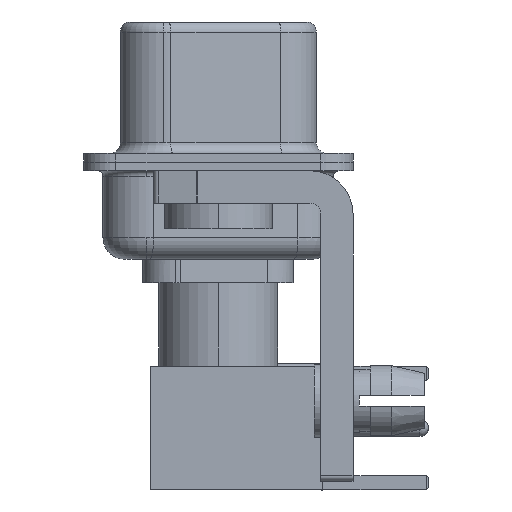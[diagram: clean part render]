
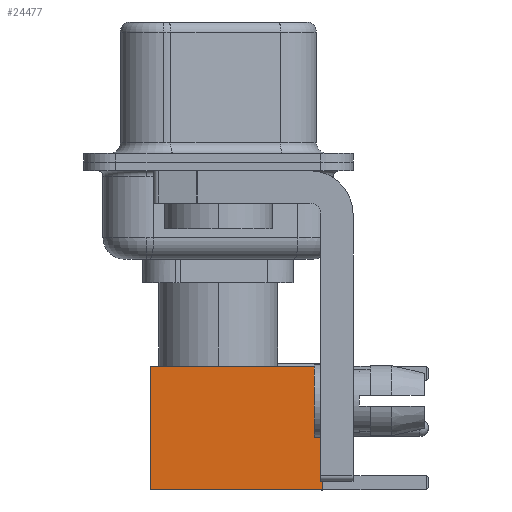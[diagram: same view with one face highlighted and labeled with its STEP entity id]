
A CAD part, left-side view. The second image highlights one B-rep face of the part: STEP entity #24477.
In plain terms, the highlighted face is planar.
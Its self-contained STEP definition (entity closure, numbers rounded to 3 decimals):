
#1158 = DIRECTION ( 'NONE',  ( 0., 0., -1. ) ) ;
#1505 = DIRECTION ( 'NONE',  ( 0., 0., -1. ) ) ;
#1846 = VECTOR ( 'NONE', #1505, 1000. ) ;
#2632 = CARTESIAN_POINT ( 'NONE',  ( 0., 2.875, 8. ) ) ;
#2718 = ORIENTED_EDGE ( 'NONE', *, *, #3485, .F. ) ;
#2777 = VERTEX_POINT ( 'NONE', #31161 ) ;
#3291 = CARTESIAN_POINT ( 'NONE',  ( -2.875, 2.875, 0. ) ) ;
#3485 = EDGE_CURVE ( 'NONE', #31703, #12900, #14359, .T. ) ;
#5637 = AXIS2_PLACEMENT_3D ( 'NONE', #26461, #16487, #24105 ) ;
#7431 = EDGE_CURVE ( 'NONE', #2777, #30493, #19737, .T. ) ;
#7661 = CARTESIAN_POINT ( 'NONE',  ( 0., 2.875, 0. ) ) ;
#7755 = VECTOR ( 'NONE', #23257, 1000. ) ;
#7855 = VECTOR ( 'NONE', #1158, 1000. ) ;
#10343 = LINE ( 'NONE', #7661, #19544 ) ;
#11004 = EDGE_CURVE ( 'NONE', #30493, #12900, #10343, .T. ) ;
#11070 = FACE_OUTER_BOUND ( 'NONE', #27569, .T. ) ;
#12900 = VERTEX_POINT ( 'NONE', #3291 ) ;
#14359 = LINE ( 'NONE', #21275, #7855 ) ;
#16487 = DIRECTION ( 'NONE',  ( 0., 1., 0. ) ) ;
#18665 = ORIENTED_EDGE ( 'NONE', *, *, #7431, .T. ) ;
#19238 = ORIENTED_EDGE ( 'NONE', *, *, #11004, .T. ) ;
#19544 = VECTOR ( 'NONE', #25923, 1000. ) ;
#19737 = LINE ( 'NONE', #30080, #1846 ) ;
#21275 = CARTESIAN_POINT ( 'NONE',  ( -2.875, 2.875, 0. ) ) ;
#22756 = LINE ( 'NONE', #2632, #7755 ) ;
#23257 = DIRECTION ( 'NONE',  ( -1., 0., 0. ) ) ;
#23763 = PLANE ( 'NONE',  #5637 ) ;
#24105 = DIRECTION ( 'NONE',  ( 0., 0., 1. ) ) ;
#24365 = EDGE_CURVE ( 'NONE', #2777, #31703, #22756, .T. ) ;
#24477 = ADVANCED_FACE ( 'NONE', ( #11070 ), #23763, .T. ) ;
#25923 = DIRECTION ( 'NONE',  ( -1., 0., 0. ) ) ;
#26461 = CARTESIAN_POINT ( 'NONE',  ( 2.875, 2.875, 0. ) ) ;
#27569 = EDGE_LOOP ( 'NONE', ( #18665, #19238, #2718, #28258 ) ) ;
#28258 = ORIENTED_EDGE ( 'NONE', *, *, #24365, .F. ) ;
#28431 = CARTESIAN_POINT ( 'NONE',  ( 2.875, 2.875, 0. ) ) ;
#30080 = CARTESIAN_POINT ( 'NONE',  ( 2.875, 2.875, 0. ) ) ;
#30493 = VERTEX_POINT ( 'NONE', #28431 ) ;
#30651 = CARTESIAN_POINT ( 'NONE',  ( -2.875, 2.875, 8. ) ) ;
#31161 = CARTESIAN_POINT ( 'NONE',  ( 2.875, 2.875, 8. ) ) ;
#31703 = VERTEX_POINT ( 'NONE', #30651 ) ;
